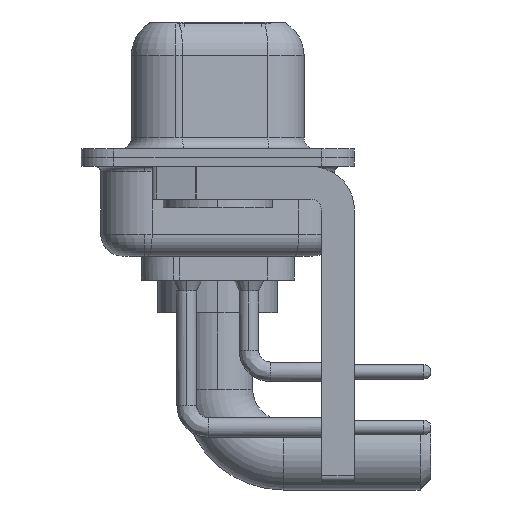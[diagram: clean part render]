
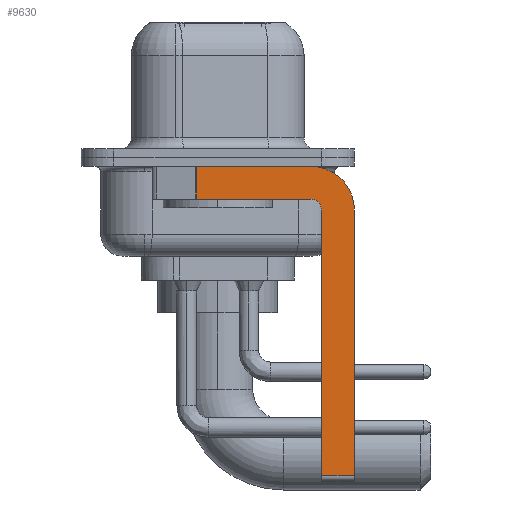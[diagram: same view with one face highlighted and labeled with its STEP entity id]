
A CAD part, left-side view. The second image highlights one B-rep face of the part: STEP entity #9630.
In plain terms, the highlighted planar face has unit normal (-1, 0, 0).
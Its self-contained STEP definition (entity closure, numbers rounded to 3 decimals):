
#796 = AXIS2_PLACEMENT_3D ( 'NONE', #3239, #17699, #22915 ) ;
#810 = DIRECTION ( 'NONE',  ( 0., 0., -1. ) ) ;
#1102 = ORIENTED_EDGE ( 'NONE', *, *, #10167, .T. ) ;
#1244 = LINE ( 'NONE', #17354, #21970 ) ;
#2629 = LINE ( 'NONE', #16975, #22807 ) ;
#2721 = DIRECTION ( 'NONE',  ( 0., 1., 0. ) ) ;
#2936 = ORIENTED_EDGE ( 'NONE', *, *, #17306, .F. ) ;
#3239 = CARTESIAN_POINT ( 'NONE',  ( -2.9, -4.25, -2.4 ) ) ;
#3350 = EDGE_CURVE ( 'NONE', #14987, #10706, #22144, .T. ) ;
#3872 = CARTESIAN_POINT ( 'NONE',  ( -2.9, -4.25, -1.9 ) ) ;
#3970 = EDGE_CURVE ( 'NONE', #15184, #10706, #15595, .T. ) ;
#4035 = CARTESIAN_POINT ( 'NONE',  ( -2.9, -4.75, -2.4 ) ) ;
#4240 = CARTESIAN_POINT ( 'NONE',  ( -2.9, -6.25, -2.4 ) ) ;
#4624 = CARTESIAN_POINT ( 'NONE',  ( -2.9, -4.25, -2.4 ) ) ;
#4712 = LINE ( 'NONE', #17287, #22064 ) ;
#6074 = DIRECTION ( 'NONE',  ( 0., -1., 0. ) ) ;
#6550 = VERTEX_POINT ( 'NONE', #23369 ) ;
#7333 = AXIS2_PLACEMENT_3D ( 'NONE', #4624, #15539, #19215 ) ;
#8069 = LINE ( 'NONE', #8419, #21637 ) ;
#8205 = CARTESIAN_POINT ( 'NONE',  ( -2.9, -6.25, -2.4 ) ) ;
#8288 = DIRECTION ( 'NONE',  ( 0., 0., -1. ) ) ;
#8419 = CARTESIAN_POINT ( 'NONE',  ( -2.9, 0.978, -1.9 ) ) ;
#9131 = VERTEX_POINT ( 'NONE', #3872 ) ;
#9511 = EDGE_CURVE ( 'NONE', #10710, #13247, #2629, .T. ) ;
#9531 = CARTESIAN_POINT ( 'NONE',  ( -2.9, -4.25, -2.4 ) ) ;
#9630 = ADVANCED_FACE ( 'NONE', ( #15203 ), #13083, .F. ) ;
#10132 = EDGE_CURVE ( 'NONE', #9131, #6550, #4712, .T. ) ;
#10167 = EDGE_CURVE ( 'NONE', #10710, #6550, #8069, .T. ) ;
#10396 = DIRECTION ( 'NONE',  ( 0., 0., 1. ) ) ;
#10675 = ORIENTED_EDGE ( 'NONE', *, *, #9511, .F. ) ;
#10706 = VERTEX_POINT ( 'NONE', #22941 ) ;
#10710 = VERTEX_POINT ( 'NONE', #17504 ) ;
#11692 = DIRECTION ( 'NONE',  ( 0., -1., 0. ) ) ;
#12412 = ORIENTED_EDGE ( 'NONE', *, *, #10132, .F. ) ;
#12897 = EDGE_CURVE ( 'NONE', #21091, #9131, #18672, .T. ) ;
#13083 = PLANE ( 'NONE',  #20553 ) ;
#13247 = VERTEX_POINT ( 'NONE', #23134 ) ;
#14158 = ORIENTED_EDGE ( 'NONE', *, *, #12897, .F. ) ;
#14855 = DIRECTION ( 'NONE',  ( 0., 0., -1. ) ) ;
#14987 = VERTEX_POINT ( 'NONE', #8205 ) ;
#15184 = VERTEX_POINT ( 'NONE', #18659 ) ;
#15203 = FACE_OUTER_BOUND ( 'NONE', #22204, .T. ) ;
#15539 = DIRECTION ( 'NONE',  ( -1., 0., 0. ) ) ;
#15595 = LINE ( 'NONE', #22818, #16759 ) ;
#15759 = ORIENTED_EDGE ( 'NONE', *, *, #23178, .F. ) ;
#15783 = ORIENTED_EDGE ( 'NONE', *, *, #3350, .F. ) ;
#16759 = VECTOR ( 'NONE', #11692, 1000. ) ;
#16975 = CARTESIAN_POINT ( 'NONE',  ( -2.9, 3., -0.4 ) ) ;
#17287 = CARTESIAN_POINT ( 'NONE',  ( -2.9, -4.25, -1.9 ) ) ;
#17306 = EDGE_CURVE ( 'NONE', #13247, #14987, #18215, .T. ) ;
#17354 = CARTESIAN_POINT ( 'NONE',  ( -2.9, -4.75, -14.8 ) ) ;
#17504 = CARTESIAN_POINT ( 'NONE',  ( -2.9, 0.978, -0.4 ) ) ;
#17699 = DIRECTION ( 'NONE',  ( 1., 0., 0. ) ) ;
#18215 = CIRCLE ( 'NONE', #796, 2. ) ;
#18659 = CARTESIAN_POINT ( 'NONE',  ( -2.9, -4.75, -14.55 ) ) ;
#18672 = CIRCLE ( 'NONE', #7333, 0.5 ) ;
#19215 = DIRECTION ( 'NONE',  ( 0., 0., 1. ) ) ;
#19224 = VECTOR ( 'NONE', #810, 1000. ) ;
#20553 = AXIS2_PLACEMENT_3D ( 'NONE', #9531, #22537, #14855 ) ;
#20941 = ORIENTED_EDGE ( 'NONE', *, *, #3970, .T. ) ;
#21091 = VERTEX_POINT ( 'NONE', #4035 ) ;
#21637 = VECTOR ( 'NONE', #8288, 1000. ) ;
#21970 = VECTOR ( 'NONE', #10396, 1000. ) ;
#22064 = VECTOR ( 'NONE', #2721, 1000. ) ;
#22144 = LINE ( 'NONE', #4240, #19224 ) ;
#22204 = EDGE_LOOP ( 'NONE', ( #10675, #1102, #12412, #14158, #15759, #20941, #15783, #2936 ) ) ;
#22537 = DIRECTION ( 'NONE',  ( 1., 0., 0. ) ) ;
#22807 = VECTOR ( 'NONE', #6074, 1000. ) ;
#22818 = CARTESIAN_POINT ( 'NONE',  ( -2.9, -4.25, -14.55 ) ) ;
#22915 = DIRECTION ( 'NONE',  ( 0., 0., -1. ) ) ;
#22941 = CARTESIAN_POINT ( 'NONE',  ( -2.9, -6.25, -14.55 ) ) ;
#23134 = CARTESIAN_POINT ( 'NONE',  ( -2.9, -4.25, -0.4 ) ) ;
#23178 = EDGE_CURVE ( 'NONE', #15184, #21091, #1244, .T. ) ;
#23369 = CARTESIAN_POINT ( 'NONE',  ( -2.9, 0.978, -1.9 ) ) ;
